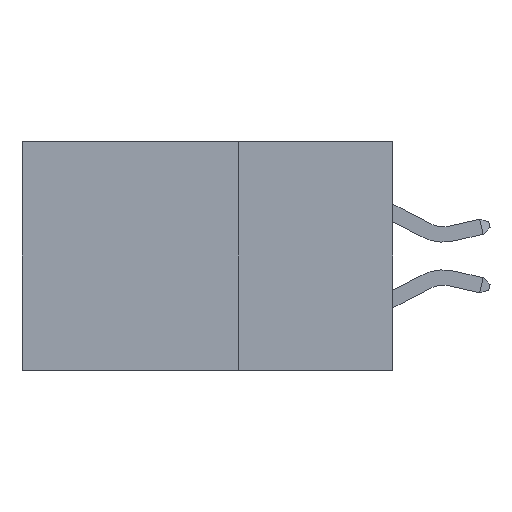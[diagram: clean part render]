
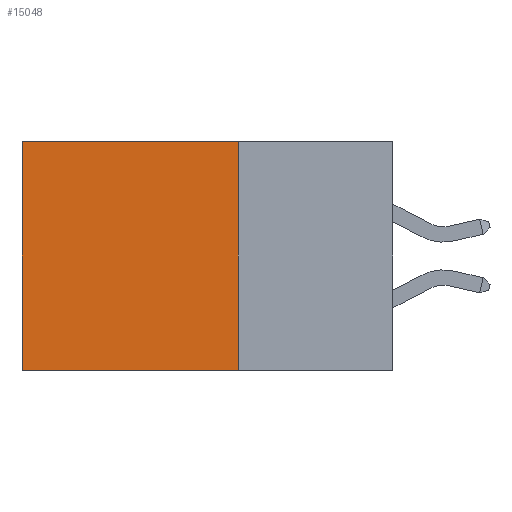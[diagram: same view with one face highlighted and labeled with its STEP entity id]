
A CAD part, left-side view. The second image highlights one B-rep face of the part: STEP entity #15048.
In plain terms, the highlighted planar face has unit normal (-1, 0, 0).
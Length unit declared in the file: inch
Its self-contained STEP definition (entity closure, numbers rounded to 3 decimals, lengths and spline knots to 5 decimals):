
#301 = CARTESIAN_POINT ( 'NONE',  ( 0.2875, 0.6, 0. ) ) ;
#849 = VECTOR ( 'NONE', #9317, 39.37008 ) ;
#905 = CARTESIAN_POINT ( 'NONE',  ( 0.2875, 0.25, 0. ) ) ;
#1094 = CARTESIAN_POINT ( 'NONE',  ( 0.2875, 0.25, -0.37 ) ) ;
#1106 = CARTESIAN_POINT ( 'NONE',  ( 0.2875, 0.6, -0.37 ) ) ;
#1451 = LINE ( 'NONE', #9340, #849 ) ;
#1872 = CARTESIAN_POINT ( 'NONE',  ( 0.2875, 0.25, 0. ) ) ;
#2328 = VERTEX_POINT ( 'NONE', #14451 ) ;
#2375 = LINE ( 'NONE', #905, #11957 ) ;
#3147 = VECTOR ( 'NONE', #14090, 39.37008 ) ;
#3221 = ORIENTED_EDGE ( 'NONE', *, *, #11982, .F. ) ;
#4179 = EDGE_CURVE ( 'NONE', #20890, #7907, #1451, .T. ) ;
#4229 = CARTESIAN_POINT ( 'NONE',  ( 0.2875, 0.25, -0.37 ) ) ;
#5346 = CARTESIAN_POINT ( 'NONE',  ( 0.2875, 0.25, 0. ) ) ;
#7907 = VERTEX_POINT ( 'NONE', #1106 ) ;
#9063 = FACE_OUTER_BOUND ( 'NONE', #19494, .T. ) ;
#9293 = DIRECTION ( 'NONE',  ( 0., 0., -1. ) ) ;
#9317 = DIRECTION ( 'NONE',  ( 0., 0., -1. ) ) ;
#9340 = CARTESIAN_POINT ( 'NONE',  ( 0.2875, 0.6, 0. ) ) ;
#10418 = ORIENTED_EDGE ( 'NONE', *, *, #16552, .T. ) ;
#11258 = LINE ( 'NONE', #1094, #15798 ) ;
#11957 = VECTOR ( 'NONE', #13495, 39.37008 ) ;
#11982 = EDGE_CURVE ( 'NONE', #2328, #12978, #21121, .T. ) ;
#12144 = ORIENTED_EDGE ( 'NONE', *, *, #4179, .T. ) ;
#12168 = ORIENTED_EDGE ( 'NONE', *, *, #19967, .F. ) ;
#12978 = VERTEX_POINT ( 'NONE', #4229 ) ;
#13495 = DIRECTION ( 'NONE',  ( 0., 1., 0. ) ) ;
#13662 = DIRECTION ( 'NONE',  ( 0., 1., 0. ) ) ;
#14090 = DIRECTION ( 'NONE',  ( 0., 0., -1. ) ) ;
#14451 = CARTESIAN_POINT ( 'NONE',  ( 0.2875, 0.25, 0. ) ) ;
#15048 = ADVANCED_FACE ( 'NONE', ( #9063 ), #16076, .F. ) ;
#15798 = VECTOR ( 'NONE', #13662, 39.37008 ) ;
#16076 = PLANE ( 'NONE',  #18691 ) ;
#16552 = EDGE_CURVE ( 'NONE', #2328, #20890, #2375, .T. ) ;
#18691 = AXIS2_PLACEMENT_3D ( 'NONE', #1872, #19454, #9293 ) ;
#19454 = DIRECTION ( 'NONE',  ( 1., 0., 0. ) ) ;
#19494 = EDGE_LOOP ( 'NONE', ( #12144, #12168, #3221, #10418 ) ) ;
#19967 = EDGE_CURVE ( 'NONE', #12978, #7907, #11258, .T. ) ;
#20890 = VERTEX_POINT ( 'NONE', #301 ) ;
#21121 = LINE ( 'NONE', #5346, #3147 ) ;
